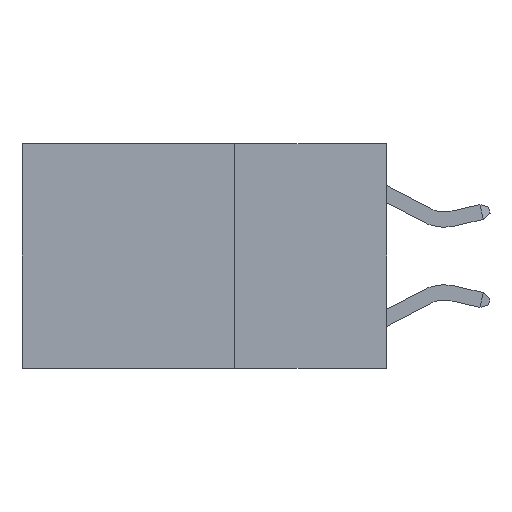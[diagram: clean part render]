
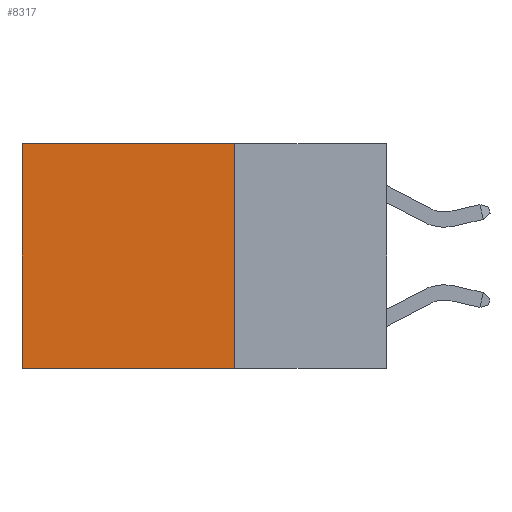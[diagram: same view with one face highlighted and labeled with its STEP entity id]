
A CAD part, left-side view. The second image highlights one B-rep face of the part: STEP entity #8317.
In plain terms, the highlighted planar face has unit normal (-1, 0, 0).
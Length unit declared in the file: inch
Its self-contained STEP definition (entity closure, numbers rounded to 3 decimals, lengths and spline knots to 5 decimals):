
#678 = VERTEX_POINT ( 'NONE', #11179 ) ;
#683 = AXIS2_PLACEMENT_3D ( 'NONE', #1951, #2851, #9133 ) ;
#1129 = CARTESIAN_POINT ( 'NONE',  ( 0.2625, 0.25, -0.37 ) ) ;
#1507 = LINE ( 'NONE', #1129, #10436 ) ;
#1951 = CARTESIAN_POINT ( 'NONE',  ( 0.2625, 0.25, 0. ) ) ;
#2099 = FACE_OUTER_BOUND ( 'NONE', #10442, .T. ) ;
#2851 = DIRECTION ( 'NONE',  ( 1., 0., 0. ) ) ;
#2876 = ORIENTED_EDGE ( 'NONE', *, *, #7237, .F. ) ;
#2913 = DIRECTION ( 'NONE',  ( 0., 0., -1. ) ) ;
#4003 = ORIENTED_EDGE ( 'NONE', *, *, #7348, .T. ) ;
#4281 = VECTOR ( 'NONE', #6112, 39.37008 ) ;
#5364 = DIRECTION ( 'NONE',  ( 0., 0., -1. ) ) ;
#5465 = VECTOR ( 'NONE', #2913, 39.37008 ) ;
#6112 = DIRECTION ( 'NONE',  ( 0., 1., 0. ) ) ;
#6273 = CARTESIAN_POINT ( 'NONE',  ( 0.2625, 0.25, -0.37 ) ) ;
#6488 = ORIENTED_EDGE ( 'NONE', *, *, #8407, .F. ) ;
#6864 = ORIENTED_EDGE ( 'NONE', *, *, #9633, .T. ) ;
#7218 = CARTESIAN_POINT ( 'NONE',  ( 0.2625, 0.25, 0. ) ) ;
#7237 = EDGE_CURVE ( 'NONE', #10122, #8882, #10794, .T. ) ;
#7348 = EDGE_CURVE ( 'NONE', #678, #9493, #9938, .T. ) ;
#8003 = VECTOR ( 'NONE', #5364, 39.37008 ) ;
#8274 = PLANE ( 'NONE',  #683 ) ;
#8317 = ADVANCED_FACE ( 'NONE', ( #2099 ), #8274, .F. ) ;
#8407 = EDGE_CURVE ( 'NONE', #8882, #9493, #1507, .T. ) ;
#8882 = VERTEX_POINT ( 'NONE', #6273 ) ;
#9133 = DIRECTION ( 'NONE',  ( 0., 0., -1. ) ) ;
#9493 = VERTEX_POINT ( 'NONE', #10511 ) ;
#9633 = EDGE_CURVE ( 'NONE', #10122, #678, #11319, .T. ) ;
#9938 = LINE ( 'NONE', #10879, #5465 ) ;
#10122 = VERTEX_POINT ( 'NONE', #11053 ) ;
#10436 = VECTOR ( 'NONE', #10894, 39.37008 ) ;
#10442 = EDGE_LOOP ( 'NONE', ( #4003, #6488, #2876, #6864 ) ) ;
#10511 = CARTESIAN_POINT ( 'NONE',  ( 0.2625, 0.6, -0.37 ) ) ;
#10525 = CARTESIAN_POINT ( 'NONE',  ( 0.2625, 0.25, 0. ) ) ;
#10794 = LINE ( 'NONE', #7218, #8003 ) ;
#10879 = CARTESIAN_POINT ( 'NONE',  ( 0.2625, 0.6, 0. ) ) ;
#10894 = DIRECTION ( 'NONE',  ( 0., 1., 0. ) ) ;
#11053 = CARTESIAN_POINT ( 'NONE',  ( 0.2625, 0.25, 0. ) ) ;
#11179 = CARTESIAN_POINT ( 'NONE',  ( 0.2625, 0.6, 0. ) ) ;
#11319 = LINE ( 'NONE', #10525, #4281 ) ;
